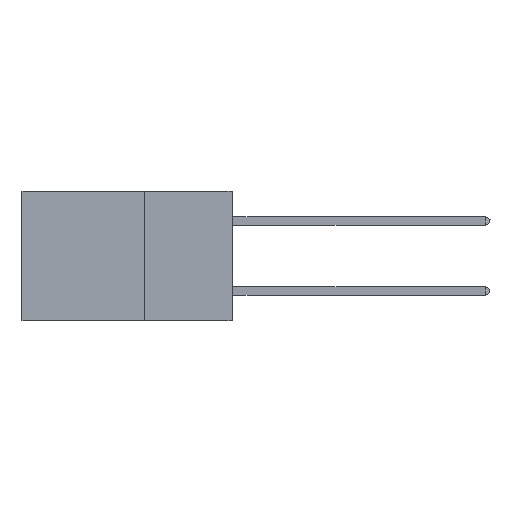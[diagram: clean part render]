
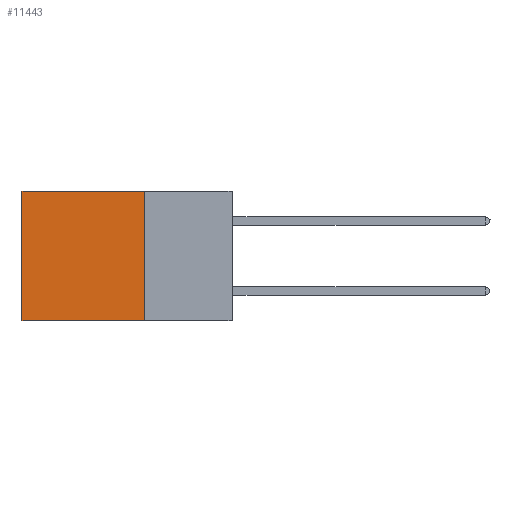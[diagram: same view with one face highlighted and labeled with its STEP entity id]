
A CAD part, left-side view. The second image highlights one B-rep face of the part: STEP entity #11443.
In plain terms, the highlighted planar face has unit normal (-1, 0, 0).
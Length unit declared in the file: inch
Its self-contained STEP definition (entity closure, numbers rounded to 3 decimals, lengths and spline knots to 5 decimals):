
#426 = ORIENTED_EDGE ( 'NONE', *, *, #24571, .T. ) ;
#575 = DIRECTION ( 'NONE',  ( 0., 1., 0. ) ) ;
#963 = CARTESIAN_POINT ( 'NONE',  ( 0.2875, 0.25, 0. ) ) ;
#1638 = VECTOR ( 'NONE', #6633, 39.37008 ) ;
#2014 = CARTESIAN_POINT ( 'NONE',  ( 0.2875, 0.6, 0. ) ) ;
#2126 = EDGE_CURVE ( 'NONE', #18142, #22886, #7374, .T. ) ;
#4647 = EDGE_CURVE ( 'NONE', #7032, #6625, #6500, .T. ) ;
#5640 = ORIENTED_EDGE ( 'NONE', *, *, #6399, .F. ) ;
#5792 = CARTESIAN_POINT ( 'NONE',  ( 0.2875, 0.25, 0. ) ) ;
#6399 = EDGE_CURVE ( 'NONE', #18142, #7032, #22482, .T. ) ;
#6500 = LINE ( 'NONE', #8345, #19116 ) ;
#6625 = VERTEX_POINT ( 'NONE', #12388 ) ;
#6633 = DIRECTION ( 'NONE',  ( 0., 0., -1. ) ) ;
#6675 = AXIS2_PLACEMENT_3D ( 'NONE', #963, #10715, #17304 ) ;
#7032 = VERTEX_POINT ( 'NONE', #20409 ) ;
#7259 = CARTESIAN_POINT ( 'NONE',  ( 0.2875, 0.25, 0. ) ) ;
#7374 = LINE ( 'NONE', #5792, #24501 ) ;
#8345 = CARTESIAN_POINT ( 'NONE',  ( 0.2875, 0.25, -0.37 ) ) ;
#9077 = EDGE_LOOP ( 'NONE', ( #426, #10755, #5640, #16003 ) ) ;
#10715 = DIRECTION ( 'NONE',  ( 1., 0., 0. ) ) ;
#10755 = ORIENTED_EDGE ( 'NONE', *, *, #4647, .F. ) ;
#11443 = ADVANCED_FACE ( 'NONE', ( #19025 ), #18890, .F. ) ;
#11726 = DIRECTION ( 'NONE',  ( 0., 1., 0. ) ) ;
#12388 = CARTESIAN_POINT ( 'NONE',  ( 0.2875, 0.6, -0.37 ) ) ;
#14741 = CARTESIAN_POINT ( 'NONE',  ( 0.2875, 0.6, 0. ) ) ;
#16003 = ORIENTED_EDGE ( 'NONE', *, *, #2126, .T. ) ;
#17117 = LINE ( 'NONE', #14741, #20316 ) ;
#17252 = DIRECTION ( 'NONE',  ( 0., 0., -1. ) ) ;
#17304 = DIRECTION ( 'NONE',  ( 0., 0., -1. ) ) ;
#18142 = VERTEX_POINT ( 'NONE', #20144 ) ;
#18890 = PLANE ( 'NONE',  #6675 ) ;
#19025 = FACE_OUTER_BOUND ( 'NONE', #9077, .T. ) ;
#19116 = VECTOR ( 'NONE', #575, 39.37008 ) ;
#20144 = CARTESIAN_POINT ( 'NONE',  ( 0.2875, 0.25, 0. ) ) ;
#20316 = VECTOR ( 'NONE', #17252, 39.37008 ) ;
#20409 = CARTESIAN_POINT ( 'NONE',  ( 0.2875, 0.25, -0.37 ) ) ;
#22482 = LINE ( 'NONE', #7259, #1638 ) ;
#22886 = VERTEX_POINT ( 'NONE', #2014 ) ;
#24501 = VECTOR ( 'NONE', #11726, 39.37008 ) ;
#24571 = EDGE_CURVE ( 'NONE', #22886, #6625, #17117, .T. ) ;
